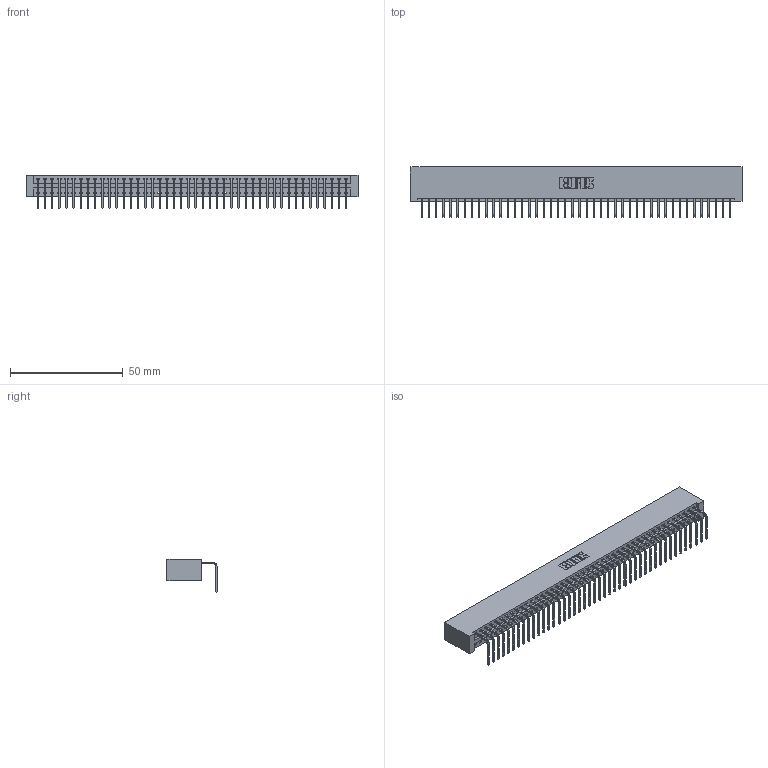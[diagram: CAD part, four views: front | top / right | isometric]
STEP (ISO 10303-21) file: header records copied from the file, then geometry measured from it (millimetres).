
FILE_DESCRIPTION (( 'STEP AP203' ), '1' );
FILE_NAME ('396-044-558-101.STEP', '2019-11-01T08:04:46', ( '' ), ( '' ), 'SwSTEP 2.0', 'SolidWorks 2016', '' );
FILE_SCHEMA (( 'CONFIG_CONTROL_DESIGN' ));
Length unit declared in the file: inch
Products named in the file (3): 345-292-001_558 Tail - 2; 396-044-558-101; 346 Part_No Mounting Lugs
Assembly tree (45 placements, depth 2):
  396-044-558-101
    346 Part_No Mounting Lugs
    345-292-001_558 Tail - 2  x44
Bounding box: 146.94 x 22.16 x 14.73 mm (x, y, z)
Volume: 14775.1 mm3; surface area: 19438.2 mm2
Topology: 45 solids, 45 shells, 2754 faces, 8313 edges, 5482 vertices
Faces by surface type: plane 1920, cylinder 834
Entity records: 26845 total; most frequent: CARTESIAN_POINT 4608, ORIENTED_EDGE 4586, DIRECTION 4057, EDGE_CURVE 2293, LINE 1993, VECTOR 1993, VERTEX_POINT 1526, AXIS2_PLACEMENT_3D 1032
